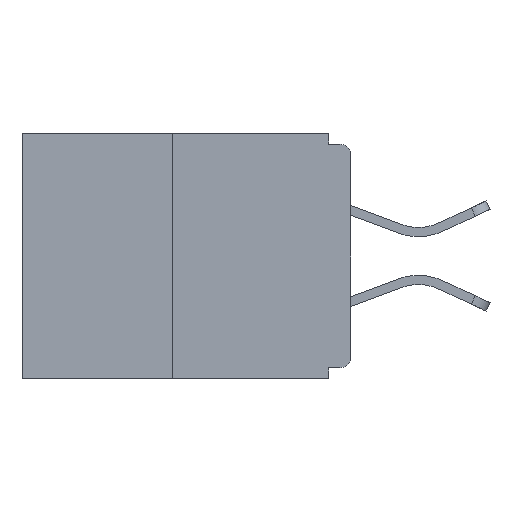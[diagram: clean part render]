
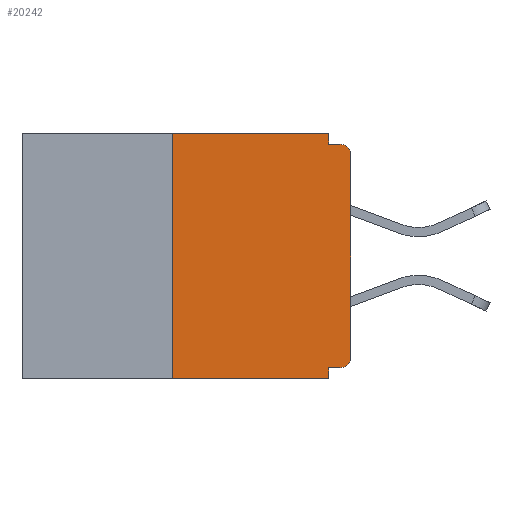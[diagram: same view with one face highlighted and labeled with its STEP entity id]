
A CAD part, left-side view. The second image highlights one B-rep face of the part: STEP entity #20242.
In plain terms, the highlighted planar face has unit normal (-1, 0, 0).
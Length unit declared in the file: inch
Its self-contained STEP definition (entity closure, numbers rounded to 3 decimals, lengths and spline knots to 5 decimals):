
#627 = VECTOR ( 'NONE', #2227, 39.37008 ) ;
#1125 = CARTESIAN_POINT ( 'NONE',  ( 0., 0.031, -0.343 ) ) ;
#1416 = VERTEX_POINT ( 'NONE', #21362 ) ;
#1658 = DIRECTION ( 'NONE',  ( 0., 0., -1. ) ) ;
#1947 = VECTOR ( 'NONE', #14515, 39.37008 ) ;
#2227 = DIRECTION ( 'NONE',  ( 0., 0., -1. ) ) ;
#2419 = DIRECTION ( 'NONE',  ( 0., 0., -1. ) ) ;
#2420 = LINE ( 'NONE', #13955, #8092 ) ;
#2574 = AXIS2_PLACEMENT_3D ( 'NONE', #7890, #7241, #1658 ) ;
#3117 = EDGE_CURVE ( 'NONE', #8508, #18584, #3983, .T. ) ;
#3446 = ORIENTED_EDGE ( 'NONE', *, *, #14019, .F. ) ;
#3983 = LINE ( 'NONE', #9857, #23151 ) ;
#4312 = CARTESIAN_POINT ( 'NONE',  ( 0., 0.031, 0. ) ) ;
#4323 = VECTOR ( 'NONE', #5380, 39.37008 ) ;
#4428 = DIRECTION ( 'NONE',  ( 0., 0., 1. ) ) ;
#5380 = DIRECTION ( 'NONE',  ( 0., 0., 1. ) ) ;
#5805 = VECTOR ( 'NONE', #4428, 39.37008 ) ;
#6113 = CARTESIAN_POINT ( 'NONE',  ( 0., 0., -0.313 ) ) ;
#6472 = CARTESIAN_POINT ( 'NONE',  ( 0., 0.46, 0. ) ) ;
#7241 = DIRECTION ( 'NONE',  ( -1., 0., 0. ) ) ;
#7520 = CIRCLE ( 'NONE', #2574, 0.015 ) ;
#7760 = DIRECTION ( 'NONE',  ( 0., 0., -1. ) ) ;
#7890 = CARTESIAN_POINT ( 'NONE',  ( 0., 0.015, -0.313 ) ) ;
#8092 = VECTOR ( 'NONE', #14119, 39.37008 ) ;
#8508 = VERTEX_POINT ( 'NONE', #4312 ) ;
#9110 = VERTEX_POINT ( 'NONE', #6113 ) ;
#9181 = DIRECTION ( 'NONE',  ( 0., 0., -1. ) ) ;
#9345 = PLANE ( 'NONE',  #20958 ) ;
#9648 = CARTESIAN_POINT ( 'NONE',  ( 0., 0.46, -0.343 ) ) ;
#9772 = DIRECTION ( 'NONE',  ( -1., 0., 0. ) ) ;
#9857 = CARTESIAN_POINT ( 'NONE',  ( 0., 0.031, 0. ) ) ;
#10029 = CARTESIAN_POINT ( 'NONE',  ( 0., 0., 0. ) ) ;
#10095 = ORIENTED_EDGE ( 'NONE', *, *, #13873, .T. ) ;
#10246 = ORIENTED_EDGE ( 'NONE', *, *, #16054, .T. ) ;
#10809 = VERTEX_POINT ( 'NONE', #10929 ) ;
#10856 = LINE ( 'NONE', #6472, #23736 ) ;
#10908 = EDGE_CURVE ( 'NONE', #15836, #1416, #19970, .T. ) ;
#10929 = CARTESIAN_POINT ( 'NONE',  ( 0., 0.015, -0.328 ) ) ;
#11104 = LINE ( 'NONE', #9648, #21848 ) ;
#11502 = CARTESIAN_POINT ( 'NONE',  ( 0., 0.25, 0. ) ) ;
#11660 = ORIENTED_EDGE ( 'NONE', *, *, #3117, .F. ) ;
#11822 = LINE ( 'NONE', #15214, #4323 ) ;
#11877 = CARTESIAN_POINT ( 'NONE',  ( 0., 0.015, -0.03 ) ) ;
#12048 = EDGE_CURVE ( 'NONE', #18972, #13292, #11822, .T. ) ;
#12062 = CARTESIAN_POINT ( 'NONE',  ( 0., 0.25, -0.343 ) ) ;
#12272 = EDGE_CURVE ( 'NONE', #9110, #15836, #19898, .T. ) ;
#12390 = EDGE_CURVE ( 'NONE', #18584, #1416, #12742, .T. ) ;
#12539 = VERTEX_POINT ( 'NONE', #14937 ) ;
#12742 = LINE ( 'NONE', #18432, #1947 ) ;
#13020 = ORIENTED_EDGE ( 'NONE', *, *, #10908, .T. ) ;
#13061 = DIRECTION ( 'NONE',  ( 1., 0., 0. ) ) ;
#13292 = VERTEX_POINT ( 'NONE', #11502 ) ;
#13459 = ORIENTED_EDGE ( 'NONE', *, *, #15263, .F. ) ;
#13873 = EDGE_CURVE ( 'NONE', #10809, #9110, #7520, .T. ) ;
#13955 = CARTESIAN_POINT ( 'NONE',  ( 0., 0., -0.328 ) ) ;
#14019 = EDGE_CURVE ( 'NONE', #12539, #18436, #23999, .T. ) ;
#14070 = ORIENTED_EDGE ( 'NONE', *, *, #12272, .T. ) ;
#14097 = ORIENTED_EDGE ( 'NONE', *, *, #12390, .F. ) ;
#14119 = DIRECTION ( 'NONE',  ( 0., 1., 0. ) ) ;
#14515 = DIRECTION ( 'NONE',  ( 0., -1., 0. ) ) ;
#14937 = CARTESIAN_POINT ( 'NONE',  ( 0., 0.031, -0.328 ) ) ;
#15063 = DIRECTION ( 'NONE',  ( 0., -1., 0. ) ) ;
#15214 = CARTESIAN_POINT ( 'NONE',  ( 0., 0.25, 0. ) ) ;
#15263 = EDGE_CURVE ( 'NONE', #13292, #8508, #10856, .T. ) ;
#15729 = FACE_OUTER_BOUND ( 'NONE', #17882, .T. ) ;
#15836 = VERTEX_POINT ( 'NONE', #23903 ) ;
#15952 = EDGE_CURVE ( 'NONE', #10809, #12539, #2420, .T. ) ;
#16054 = EDGE_CURVE ( 'NONE', #18972, #18436, #11104, .T. ) ;
#17882 = EDGE_LOOP ( 'NONE', ( #13459, #19105, #10246, #3446, #17965, #10095, #14070, #13020, #14097, #11660 ) ) ;
#17965 = ORIENTED_EDGE ( 'NONE', *, *, #15952, .F. ) ;
#18432 = CARTESIAN_POINT ( 'NONE',  ( 0., 0., -0.015 ) ) ;
#18436 = VERTEX_POINT ( 'NONE', #1125 ) ;
#18584 = VERTEX_POINT ( 'NONE', #24392 ) ;
#18972 = VERTEX_POINT ( 'NONE', #12062 ) ;
#19105 = ORIENTED_EDGE ( 'NONE', *, *, #12048, .F. ) ;
#19637 = CARTESIAN_POINT ( 'NONE',  ( 0., 0.031, -0.343 ) ) ;
#19740 = DIRECTION ( 'NONE',  ( 0., -1., 0. ) ) ;
#19898 = LINE ( 'NONE', #10029, #5805 ) ;
#19970 = CIRCLE ( 'NONE', #23081, 0.015 ) ;
#20242 = ADVANCED_FACE ( 'NONE', ( #15729 ), #9345, .F. ) ;
#20657 = CARTESIAN_POINT ( 'NONE',  ( 0., 0.46, 0. ) ) ;
#20958 = AXIS2_PLACEMENT_3D ( 'NONE', #20657, #13061, #9181 ) ;
#21362 = CARTESIAN_POINT ( 'NONE',  ( 0., 0.015, -0.015 ) ) ;
#21848 = VECTOR ( 'NONE', #15063, 39.37008 ) ;
#23081 = AXIS2_PLACEMENT_3D ( 'NONE', #11877, #9772, #7760 ) ;
#23151 = VECTOR ( 'NONE', #2419, 39.37008 ) ;
#23736 = VECTOR ( 'NONE', #19740, 39.37008 ) ;
#23903 = CARTESIAN_POINT ( 'NONE',  ( 0., 0., -0.03 ) ) ;
#23999 = LINE ( 'NONE', #19637, #627 ) ;
#24392 = CARTESIAN_POINT ( 'NONE',  ( 0., 0.031, -0.015 ) ) ;
